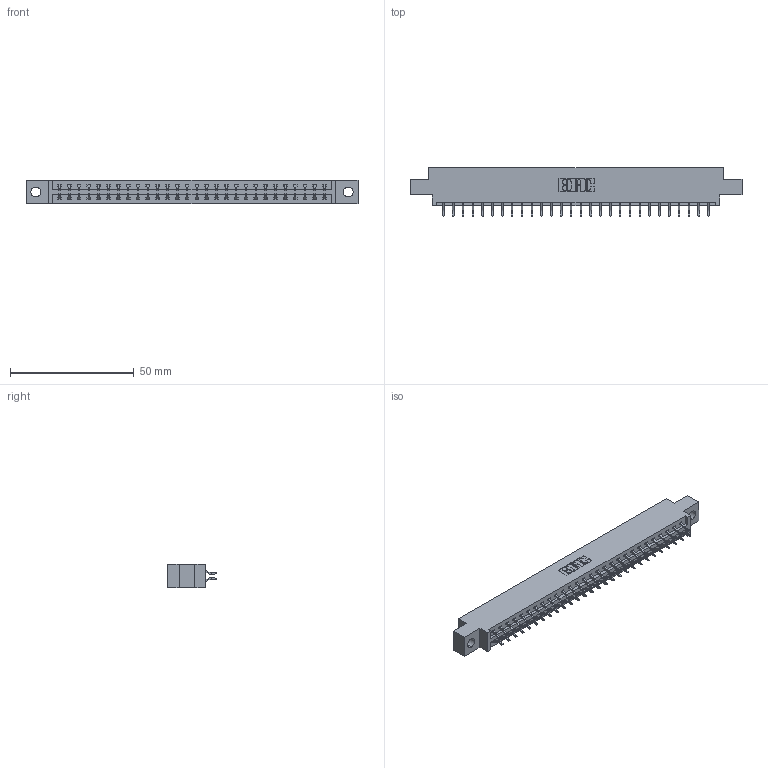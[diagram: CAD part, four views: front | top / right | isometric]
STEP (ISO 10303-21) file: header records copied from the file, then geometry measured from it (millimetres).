
FILE_DESCRIPTION (( 'STEP AP203' ), '1' );
FILE_NAME ('337-056-556-804.STEP', '2018-08-10T03:44:56', ( '' ), ( '' ), 'SwSTEP 2.0', 'SolidWorks 2016', '' );
FILE_SCHEMA (( 'CONFIG_CONTROL_DESIGN' ));
Length unit declared in the file: inch
Products named in the file (3): 337 Part_0.170 Offset - 0.156 Dia-TH; 345-292-001_556 Tail; 337-056-556-804
Assembly tree (57 placements, depth 2):
  337-056-556-804
    337 Part_0.170 Offset - 0.156 Dia-TH
    345-292-001_556 Tail  x56
Bounding box: 133.96 x 19.57 x 9.4 mm (x, y, z)
Volume: 13723.8 mm3; surface area: 15224.9 mm2
Topology: 57 solids, 57 shells, 3478 faces, 10347 edges, 6822 vertices
Faces by surface type: plane 2426, cylinder 1052
Entity records: 23875 total; most frequent: CARTESIAN_POINT 4050, ORIENTED_EDGE 3974, DIRECTION 3459, EDGE_CURVE 1987, LINE 1851, VECTOR 1851, VERTEX_POINT 1322, AXIS2_PLACEMENT_3D 804
